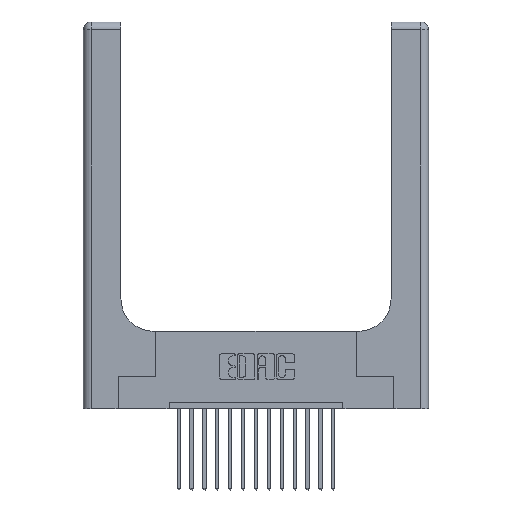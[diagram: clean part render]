
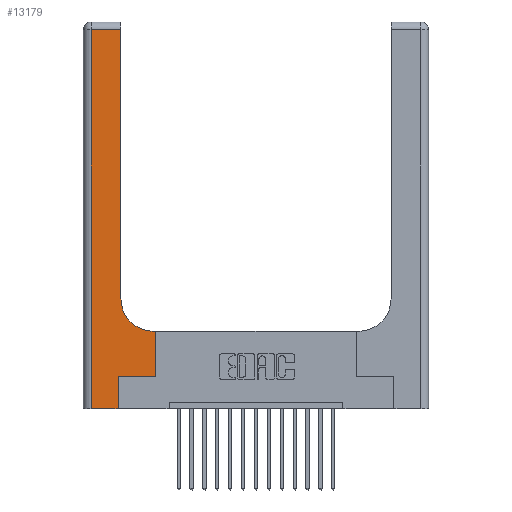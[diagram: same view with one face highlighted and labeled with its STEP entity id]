
A CAD part, top view. The second image highlights one B-rep face of the part: STEP entity #13179.
In plain terms, the highlighted planar face has unit normal (0, 0, 1).
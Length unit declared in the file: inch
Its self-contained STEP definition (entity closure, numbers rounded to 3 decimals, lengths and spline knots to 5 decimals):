
#354 = VECTOR ( 'NONE', #10283, 39.37008 ) ;
#798 = VERTEX_POINT ( 'NONE', #10021 ) ;
#1139 = CARTESIAN_POINT ( 'NONE',  ( 0.269, 0.25, 0.37 ) ) ;
#1620 = ORIENTED_EDGE ( 'NONE', *, *, #14123, .T. ) ;
#1873 = VECTOR ( 'NONE', #4060, 39.37008 ) ;
#2591 = DIRECTION ( 'NONE',  ( 1., 0., 0. ) ) ;
#2613 = CARTESIAN_POINT ( 'NONE',  ( 0., 2.94, 0.37 ) ) ;
#2711 = VERTEX_POINT ( 'NONE', #3866 ) ;
#2880 = VECTOR ( 'NONE', #2591, 39.37008 ) ;
#3031 = CARTESIAN_POINT ( 'NONE',  ( 0.5585, 0.25, 0.37 ) ) ;
#3140 = CIRCLE ( 'NONE', #18103, 0.25 ) ;
#3353 = CARTESIAN_POINT ( 'NONE',  ( 0., 3., 0.37 ) ) ;
#3460 = EDGE_LOOP ( 'NONE', ( #12820, #16094, #4112, #7152, #13512, #18543, #18655, #9167, #1620 ) ) ;
#3866 = CARTESIAN_POINT ( 'NONE',  ( 0.5585, 0.25, 0.37 ) ) ;
#3885 = FACE_OUTER_BOUND ( 'NONE', #3460, .T. ) ;
#4060 = DIRECTION ( 'NONE',  ( 1., 0., 0. ) ) ;
#4112 = ORIENTED_EDGE ( 'NONE', *, *, #14314, .T. ) ;
#4118 = VECTOR ( 'NONE', #18700, 39.37008 ) ;
#4401 = LINE ( 'NONE', #5588, #1873 ) ;
#4675 = VERTEX_POINT ( 'NONE', #15409 ) ;
#4842 = DIRECTION ( 'NONE',  ( 0., 0., -1. ) ) ;
#5229 = CARTESIAN_POINT ( 'NONE',  ( 0.2915, 3., 0.37 ) ) ;
#5380 = VERTEX_POINT ( 'NONE', #6650 ) ;
#5588 = CARTESIAN_POINT ( 'NONE',  ( 0., 0., 0.37 ) ) ;
#6650 = CARTESIAN_POINT ( 'NONE',  ( 0.5585, 0.6, 0.37 ) ) ;
#6733 = EDGE_CURVE ( 'NONE', #798, #10842, #18728, .T. ) ;
#6765 = EDGE_CURVE ( 'NONE', #4675, #9143, #16249, .T. ) ;
#6817 = EDGE_CURVE ( 'NONE', #10842, #12942, #7106, .T. ) ;
#6883 = VECTOR ( 'NONE', #12907, 39.37008 ) ;
#6967 = VECTOR ( 'NONE', #10976, 39.37008 ) ;
#7044 = LINE ( 'NONE', #1139, #2880 ) ;
#7106 = LINE ( 'NONE', #2613, #13475 ) ;
#7152 = ORIENTED_EDGE ( 'NONE', *, *, #18438, .T. ) ;
#7770 = CARTESIAN_POINT ( 'NONE',  ( 0.5415, 0.85, 0.37 ) ) ;
#8327 = CARTESIAN_POINT ( 'NONE',  ( 0.06, 0., 0.37 ) ) ;
#9143 = VERTEX_POINT ( 'NONE', #11801 ) ;
#9167 = ORIENTED_EDGE ( 'NONE', *, *, #16709, .T. ) ;
#10021 = CARTESIAN_POINT ( 'NONE',  ( 0.2915, 0.85, 0.37 ) ) ;
#10170 = DIRECTION ( 'NONE',  ( -1., 0., 0. ) ) ;
#10283 = DIRECTION ( 'NONE',  ( 0., 1., 0. ) ) ;
#10479 = VECTOR ( 'NONE', #15215, 39.37008 ) ;
#10842 = VERTEX_POINT ( 'NONE', #12625 ) ;
#10976 = DIRECTION ( 'NONE',  ( -1., 0., 0. ) ) ;
#11602 = AXIS2_PLACEMENT_3D ( 'NONE', #3353, #4842, #12181 ) ;
#11790 = CARTESIAN_POINT ( 'NONE',  ( 0.06, 2.94, 0.37 ) ) ;
#11801 = CARTESIAN_POINT ( 'NONE',  ( 0.269, 0.25, 0.37 ) ) ;
#12124 = PLANE ( 'NONE',  #11602 ) ;
#12181 = DIRECTION ( 'NONE',  ( -1., 0., 0. ) ) ;
#12262 = DIRECTION ( 'NONE',  ( 0., 0., -1. ) ) ;
#12296 = LINE ( 'NONE', #12388, #10479 ) ;
#12388 = CARTESIAN_POINT ( 'NONE',  ( 0.06, 3., 0.37 ) ) ;
#12625 = CARTESIAN_POINT ( 'NONE',  ( 0.2915, 2.94, 0.37 ) ) ;
#12820 = ORIENTED_EDGE ( 'NONE', *, *, #6733, .T. ) ;
#12866 = EDGE_CURVE ( 'NONE', #2711, #5380, #17500, .T. ) ;
#12907 = DIRECTION ( 'NONE',  ( 0., 1., 0. ) ) ;
#12942 = VERTEX_POINT ( 'NONE', #11790 ) ;
#13179 = ADVANCED_FACE ( 'NONE', ( #3885 ), #12124, .F. ) ;
#13475 = VECTOR ( 'NONE', #10170, 39.37008 ) ;
#13512 = ORIENTED_EDGE ( 'NONE', *, *, #6765, .T. ) ;
#14123 = EDGE_CURVE ( 'NONE', #16325, #798, #3140, .T. ) ;
#14314 = EDGE_CURVE ( 'NONE', #12942, #14501, #12296, .T. ) ;
#14501 = VERTEX_POINT ( 'NONE', #8327 ) ;
#14979 = EDGE_CURVE ( 'NONE', #9143, #2711, #7044, .T. ) ;
#15185 = LINE ( 'NONE', #16734, #6967 ) ;
#15215 = DIRECTION ( 'NONE',  ( 0., -1., 0. ) ) ;
#15409 = CARTESIAN_POINT ( 'NONE',  ( 0.269, 0., 0.37 ) ) ;
#15724 = CARTESIAN_POINT ( 'NONE',  ( 0.5415, 0.6, 0.37 ) ) ;
#16094 = ORIENTED_EDGE ( 'NONE', *, *, #6817, .T. ) ;
#16249 = LINE ( 'NONE', #18336, #4118 ) ;
#16325 = VERTEX_POINT ( 'NONE', #15724 ) ;
#16709 = EDGE_CURVE ( 'NONE', #5380, #16325, #15185, .T. ) ;
#16734 = CARTESIAN_POINT ( 'NONE',  ( 0.2915, 0.6, 0.37 ) ) ;
#17500 = LINE ( 'NONE', #3031, #354 ) ;
#17950 = DIRECTION ( 'NONE',  ( 1., 0., 0. ) ) ;
#18103 = AXIS2_PLACEMENT_3D ( 'NONE', #7770, #12262, #17950 ) ;
#18336 = CARTESIAN_POINT ( 'NONE',  ( 0.269, 0., 0.37 ) ) ;
#18438 = EDGE_CURVE ( 'NONE', #14501, #4675, #4401, .T. ) ;
#18543 = ORIENTED_EDGE ( 'NONE', *, *, #14979, .T. ) ;
#18655 = ORIENTED_EDGE ( 'NONE', *, *, #12866, .T. ) ;
#18700 = DIRECTION ( 'NONE',  ( 0., 1., 0. ) ) ;
#18728 = LINE ( 'NONE', #5229, #6883 ) ;
